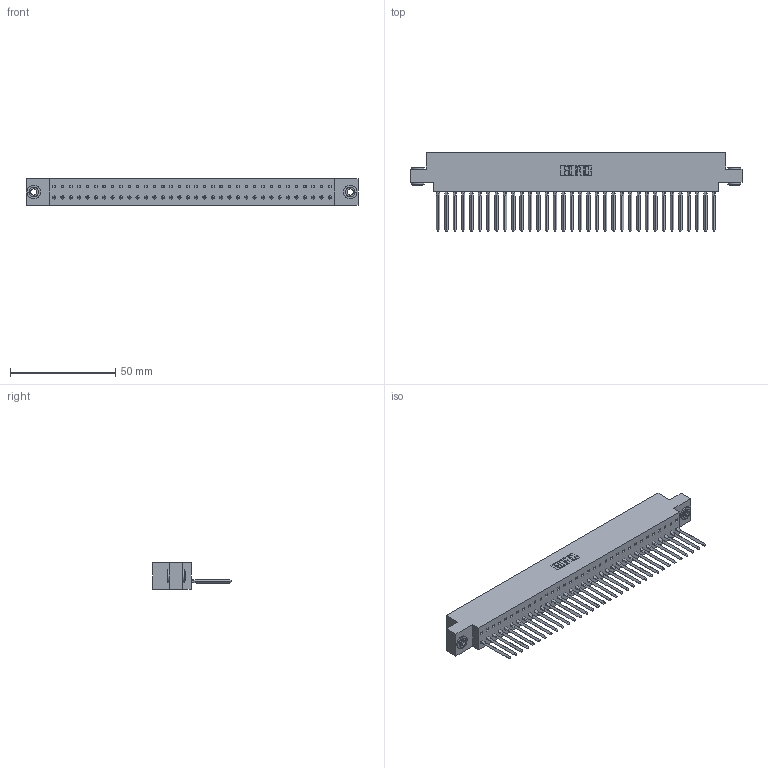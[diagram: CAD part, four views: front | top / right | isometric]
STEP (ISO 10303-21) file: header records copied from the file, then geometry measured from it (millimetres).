
FILE_DESCRIPTION (( 'STEP AP203' ), '1' );
FILE_NAME ('317-034-541-603.STEP', '2020-02-27T21:48:06', ( '' ), ( '' ), 'SwSTEP 2.0', 'SolidWorks 2016', '' );
FILE_SCHEMA (( 'CONFIG_CONTROL_DESIGN' ));
Length unit declared in the file: inch
Products named in the file (4): 317 Part_.156 Dia - TH; 317-034-541-603; 345-250-002_345-250-002-102; 317-290-002_541
Assembly tree (37 placements, depth 2):
  317-034-541-603
    317 Part_.156 Dia - TH
    317-290-002_541  x34
    345-250-002_345-250-002-102  x2
Bounding box: 157.43 x 37.34 x 12.7 mm (x, y, z)
Volume: 25303.1 mm3; surface area: 35703 mm2
Topology: 37 solids, 37 shells, 5308 faces, 15107 edges, 9818 vertices
Faces by surface type: plane 4284, cylinder 880, bspline 136, cone 8
Entity records: 51373 total; most frequent: CARTESIAN_POINT 9738, ORIENTED_EDGE 9018, DIRECTION 7443, EDGE_CURVE 4509, VECTOR 4121, LINE 4121, VERTEX_POINT 2996, AXIS2_PLACEMENT_3D 1661
